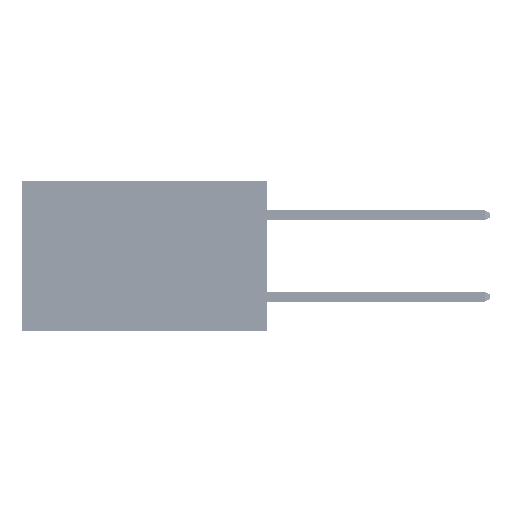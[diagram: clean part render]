
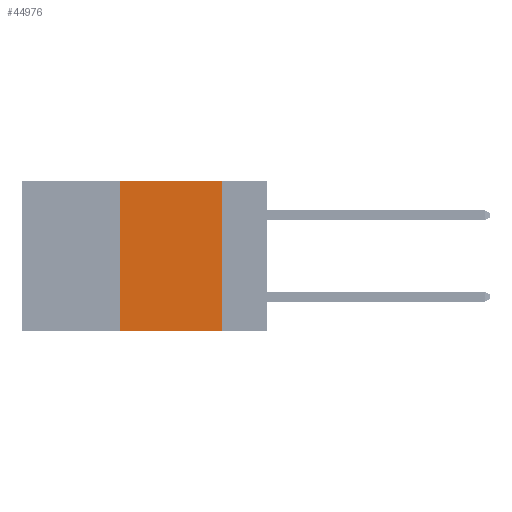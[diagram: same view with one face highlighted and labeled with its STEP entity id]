
A CAD part, left-side view. The second image highlights one B-rep face of the part: STEP entity #44976.
In plain terms, the highlighted planar face has unit normal (-1, 0, 0).
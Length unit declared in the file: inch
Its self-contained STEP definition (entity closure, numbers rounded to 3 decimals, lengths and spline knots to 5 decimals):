
#2691 = CARTESIAN_POINT ( 'NONE',  ( 0., 0.6, -0.37 ) ) ;
#3193 = CARTESIAN_POINT ( 'NONE',  ( 0., 0.11, 0. ) ) ;
#3631 = DIRECTION ( 'NONE',  ( 0., 0., 1. ) ) ;
#3890 = CARTESIAN_POINT ( 'NONE',  ( 0., 0.36, 0. ) ) ;
#4403 = DIRECTION ( 'NONE',  ( 1., 0., 0. ) ) ;
#5357 = EDGE_CURVE ( 'NONE', #50712, #13836, #35020, .T. ) ;
#5956 = EDGE_CURVE ( 'NONE', #13727, #50712, #11910, .T. ) ;
#7848 = EDGE_CURVE ( 'NONE', #13836, #14645, #30567, .T. ) ;
#8045 = DIRECTION ( 'NONE',  ( 0., 0., -1. ) ) ;
#11282 = ORIENTED_EDGE ( 'NONE', *, *, #7848, .F. ) ;
#11289 = VECTOR ( 'NONE', #22528, 39.37008 ) ;
#11910 = LINE ( 'NONE', #3890, #35116 ) ;
#13727 = VERTEX_POINT ( 'NONE', #41493 ) ;
#13836 = VERTEX_POINT ( 'NONE', #3193 ) ;
#14645 = VERTEX_POINT ( 'NONE', #44477 ) ;
#15799 = CARTESIAN_POINT ( 'NONE',  ( 0., 0.6, 0. ) ) ;
#15847 = ORIENTED_EDGE ( 'NONE', *, *, #5956, .F. ) ;
#22528 = DIRECTION ( 'NONE',  ( 0., 0., -1. ) ) ;
#26935 = CARTESIAN_POINT ( 'NONE',  ( 0., 0.11, 0. ) ) ;
#27221 = FACE_OUTER_BOUND ( 'NONE', #33760, .T. ) ;
#28932 = EDGE_CURVE ( 'NONE', #13727, #14645, #38163, .T. ) ;
#30567 = LINE ( 'NONE', #26935, #11289 ) ;
#33760 = EDGE_LOOP ( 'NONE', ( #11282, #45852, #15847, #40342 ) ) ;
#35020 = LINE ( 'NONE', #37189, #40040 ) ;
#35035 = DIRECTION ( 'NONE',  ( 0., -1., 0. ) ) ;
#35116 = VECTOR ( 'NONE', #3631, 39.37008 ) ;
#37189 = CARTESIAN_POINT ( 'NONE',  ( 0., 0.6, 0. ) ) ;
#38163 = LINE ( 'NONE', #2691, #41267 ) ;
#40040 = VECTOR ( 'NONE', #50786, 39.37008 ) ;
#40342 = ORIENTED_EDGE ( 'NONE', *, *, #28932, .T. ) ;
#41267 = VECTOR ( 'NONE', #35035, 39.37008 ) ;
#41493 = CARTESIAN_POINT ( 'NONE',  ( 0., 0.36, -0.37 ) ) ;
#43494 = PLANE ( 'NONE',  #43872 ) ;
#43498 = CARTESIAN_POINT ( 'NONE',  ( 0., 0.36, 0. ) ) ;
#43872 = AXIS2_PLACEMENT_3D ( 'NONE', #15799, #4403, #8045 ) ;
#44477 = CARTESIAN_POINT ( 'NONE',  ( 0., 0.11, -0.37 ) ) ;
#44976 = ADVANCED_FACE ( 'NONE', ( #27221 ), #43494, .F. ) ;
#45852 = ORIENTED_EDGE ( 'NONE', *, *, #5357, .F. ) ;
#50712 = VERTEX_POINT ( 'NONE', #43498 ) ;
#50786 = DIRECTION ( 'NONE',  ( 0., -1., 0. ) ) ;
